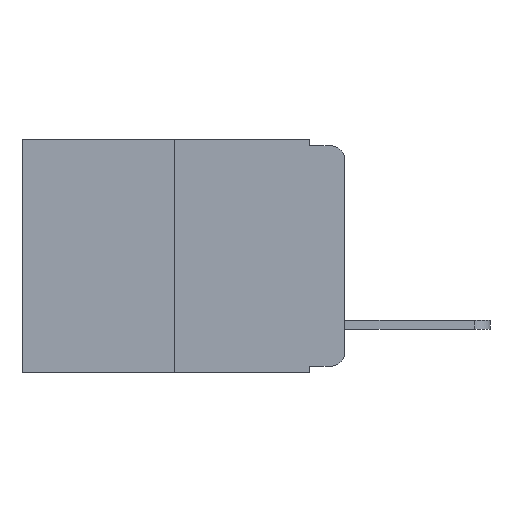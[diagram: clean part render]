
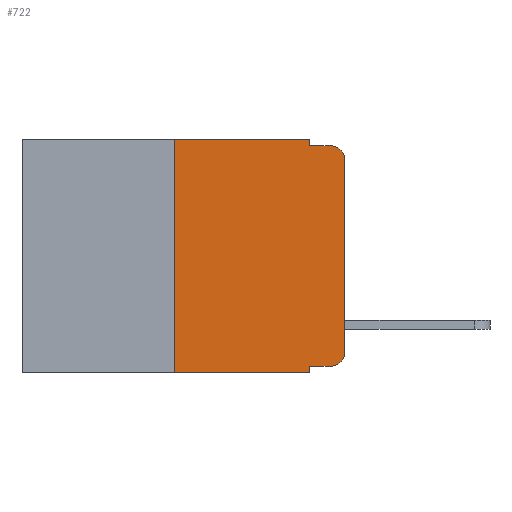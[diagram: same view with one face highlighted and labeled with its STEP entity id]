
A CAD part, left-side view. The second image highlights one B-rep face of the part: STEP entity #722.
In plain terms, the highlighted planar face has unit normal (-1, 0, 0).
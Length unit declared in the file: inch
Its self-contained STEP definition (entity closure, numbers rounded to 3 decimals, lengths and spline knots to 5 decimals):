
#90 = VERTEX_POINT ( 'NONE', #1693 ) ;
#91 = DIRECTION ( 'NONE',  ( 0., 0., -1. ) ) ;
#303 = VERTEX_POINT ( 'NONE', #9541 ) ;
#398 = CARTESIAN_POINT ( 'NONE',  ( 0., 0.051, -0.333 ) ) ;
#562 = ORIENTED_EDGE ( 'NONE', *, *, #11496, .T. ) ;
#633 = CARTESIAN_POINT ( 'NONE',  ( 0., 0.02, -0.333 ) ) ;
#647 = VERTEX_POINT ( 'NONE', #633 ) ;
#649 = EDGE_LOOP ( 'NONE', ( #9320, #9479, #10334, #10439, #10498, #10989, #1974, #3419, #3464, #562 ) ) ;
#722 = ADVANCED_FACE ( 'NONE', ( #10846 ), #858, .F. ) ;
#772 = CIRCLE ( 'NONE', #3371, 0.02 ) ;
#858 = PLANE ( 'NONE',  #11844 ) ;
#947 = VERTEX_POINT ( 'NONE', #5871 ) ;
#1477 = EDGE_CURVE ( 'NONE', #2694, #3689, #6246, .T. ) ;
#1693 = CARTESIAN_POINT ( 'NONE',  ( 0., 0.25, -0.343 ) ) ;
#1917 = DIRECTION ( 'NONE',  ( 0., 0., -1. ) ) ;
#1931 = DIRECTION ( 'NONE',  ( -1., 0., 0. ) ) ;
#1974 = ORIENTED_EDGE ( 'NONE', *, *, #8643, .T. ) ;
#1989 = CARTESIAN_POINT ( 'NONE',  ( 0., 0.02, -0.313 ) ) ;
#2170 = DIRECTION ( 'NONE',  ( 0., -1., 0. ) ) ;
#2339 = DIRECTION ( 'NONE',  ( 0., 0., -1. ) ) ;
#2387 = CIRCLE ( 'NONE', #11812, 0.02 ) ;
#2694 = VERTEX_POINT ( 'NONE', #11257 ) ;
#2844 = CARTESIAN_POINT ( 'NONE',  ( 0., 0.051, 0. ) ) ;
#3295 = DIRECTION ( 'NONE',  ( 0., -1., 0. ) ) ;
#3359 = CARTESIAN_POINT ( 'NONE',  ( 0., 0.051, -0.01 ) ) ;
#3371 = AXIS2_PLACEMENT_3D ( 'NONE', #1989, #1931, #1917 ) ;
#3419 = ORIENTED_EDGE ( 'NONE', *, *, #10983, .F. ) ;
#3464 = ORIENTED_EDGE ( 'NONE', *, *, #11152, .T. ) ;
#3556 = LINE ( 'NONE', #8826, #8219 ) ;
#3689 = VERTEX_POINT ( 'NONE', #11846 ) ;
#3952 = CARTESIAN_POINT ( 'NONE',  ( 0., 0.02, -0.01 ) ) ;
#4049 = LINE ( 'NONE', #8950, #10690 ) ;
#4551 = DIRECTION ( 'NONE',  ( 0., 0., 1. ) ) ;
#4688 = CARTESIAN_POINT ( 'NONE',  ( 0., 0.051, 0. ) ) ;
#4763 = VERTEX_POINT ( 'NONE', #3952 ) ;
#5301 = VECTOR ( 'NONE', #5320, 39.37008 ) ;
#5320 = DIRECTION ( 'NONE',  ( 0., 0., 1. ) ) ;
#5540 = DIRECTION ( 'NONE',  ( 0., 0., -1. ) ) ;
#5735 = VERTEX_POINT ( 'NONE', #398 ) ;
#5871 = CARTESIAN_POINT ( 'NONE',  ( 0., 0., -0.313 ) ) ;
#6128 = VECTOR ( 'NONE', #3295, 39.37008 ) ;
#6161 = CARTESIAN_POINT ( 'NONE',  ( 0., 0.473, 0. ) ) ;
#6246 = LINE ( 'NONE', #6362, #6128 ) ;
#6362 = CARTESIAN_POINT ( 'NONE',  ( 0., 0.473, 0. ) ) ;
#6437 = VERTEX_POINT ( 'NONE', #8781 ) ;
#7077 = CARTESIAN_POINT ( 'NONE',  ( 0., 0., 0. ) ) ;
#7108 = VECTOR ( 'NONE', #2170, 39.37008 ) ;
#7411 = VECTOR ( 'NONE', #4551, 39.37008 ) ;
#7512 = CARTESIAN_POINT ( 'NONE',  ( 0., 0.051, -0.343 ) ) ;
#7710 = LINE ( 'NONE', #7077, #7411 ) ;
#8097 = LINE ( 'NONE', #2844, #12241 ) ;
#8219 = VECTOR ( 'NONE', #8538, 39.37008 ) ;
#8360 = DIRECTION ( 'NONE',  ( 0., -1., 0. ) ) ;
#8380 = LINE ( 'NONE', #4688, #10423 ) ;
#8446 = VERTEX_POINT ( 'NONE', #7512 ) ;
#8538 = DIRECTION ( 'NONE',  ( 0., -1., 0. ) ) ;
#8603 = CARTESIAN_POINT ( 'NONE',  ( 0., 0.02, -0.03 ) ) ;
#8643 = EDGE_CURVE ( 'NONE', #90, #8446, #4049, .T. ) ;
#8781 = CARTESIAN_POINT ( 'NONE',  ( 0., 0., -0.03 ) ) ;
#8826 = CARTESIAN_POINT ( 'NONE',  ( 0., 0.051, -0.333 ) ) ;
#8900 = EDGE_CURVE ( 'NONE', #947, #6437, #7710, .T. ) ;
#8950 = CARTESIAN_POINT ( 'NONE',  ( 0., 0.473, -0.343 ) ) ;
#9087 = EDGE_CURVE ( 'NONE', #6437, #4763, #2387, .T. ) ;
#9108 = CARTESIAN_POINT ( 'NONE',  ( 0., 0.25, 0. ) ) ;
#9320 = ORIENTED_EDGE ( 'NONE', *, *, #8900, .T. ) ;
#9352 = DIRECTION ( 'NONE',  ( -1., 0., 0. ) ) ;
#9479 = ORIENTED_EDGE ( 'NONE', *, *, #9087, .T. ) ;
#9541 = CARTESIAN_POINT ( 'NONE',  ( 0., 0.051, -0.01 ) ) ;
#9902 = EDGE_CURVE ( 'NONE', #303, #4763, #11693, .T. ) ;
#10004 = EDGE_CURVE ( 'NONE', #3689, #303, #8380, .T. ) ;
#10048 = EDGE_CURVE ( 'NONE', #90, #2694, #12256, .T. ) ;
#10097 = DIRECTION ( 'NONE',  ( 0., 0., -1. ) ) ;
#10334 = ORIENTED_EDGE ( 'NONE', *, *, #9902, .F. ) ;
#10423 = VECTOR ( 'NONE', #5540, 39.37008 ) ;
#10439 = ORIENTED_EDGE ( 'NONE', *, *, #10004, .F. ) ;
#10498 = ORIENTED_EDGE ( 'NONE', *, *, #1477, .F. ) ;
#10690 = VECTOR ( 'NONE', #8360, 39.37008 ) ;
#10846 = FACE_OUTER_BOUND ( 'NONE', #649, .T. ) ;
#10983 = EDGE_CURVE ( 'NONE', #5735, #8446, #8097, .T. ) ;
#10989 = ORIENTED_EDGE ( 'NONE', *, *, #10048, .F. ) ;
#11152 = EDGE_CURVE ( 'NONE', #5735, #647, #3556, .T. ) ;
#11257 = CARTESIAN_POINT ( 'NONE',  ( 0., 0.25, 0. ) ) ;
#11496 = EDGE_CURVE ( 'NONE', #647, #947, #772, .T. ) ;
#11693 = LINE ( 'NONE', #3359, #7108 ) ;
#11764 = DIRECTION ( 'NONE',  ( 1., 0., 0. ) ) ;
#11812 = AXIS2_PLACEMENT_3D ( 'NONE', #8603, #9352, #91 ) ;
#11844 = AXIS2_PLACEMENT_3D ( 'NONE', #6161, #11764, #10097 ) ;
#11846 = CARTESIAN_POINT ( 'NONE',  ( 0., 0.051, 0. ) ) ;
#12241 = VECTOR ( 'NONE', #2339, 39.37008 ) ;
#12256 = LINE ( 'NONE', #9108, #5301 ) ;
